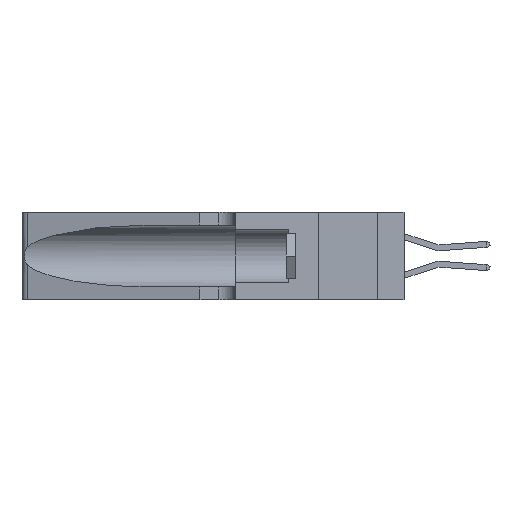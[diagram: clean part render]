
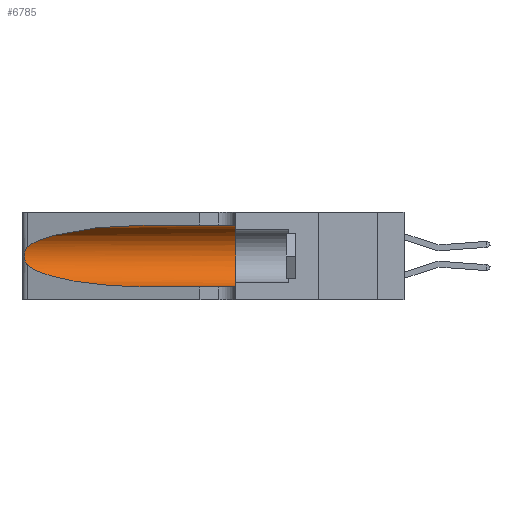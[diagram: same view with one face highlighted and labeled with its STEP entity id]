
A CAD part, left-side view. The second image highlights one B-rep face of the part: STEP entity #6785.
In plain terms, the highlighted cylindrical face has radius 3.308 mm (diameter 6.617 mm), a partial arc.
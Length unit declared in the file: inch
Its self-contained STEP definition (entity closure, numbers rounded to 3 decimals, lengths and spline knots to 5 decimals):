
#809 = ORIENTED_EDGE ( 'NONE', *, *, #11484, .T. ) ;
#860 = CARTESIAN_POINT ( 'NONE',  ( 0.1305, 0.35, 0.05475 ) ) ;
#957 = ORIENTED_EDGE ( 'NONE', *, *, #4962, .T. ) ;
#992 = DIRECTION ( 'NONE',  ( 0., -1., 0. ) ) ;
#998 = VERTEX_POINT ( 'NONE', #6603 ) ;
#1192 = DIRECTION ( 'NONE',  ( 0., 0., 1. ) ) ;
#1731 = EDGE_CURVE ( 'NONE', #15621, #19204, #7611, .T. ) ;
#1998 = CARTESIAN_POINT ( 'NONE',  ( 0.25856, 1.23593, 0.16098 ) ) ;
#2071 = CARTESIAN_POINT ( 'NONE',  ( 0.26017, 1.23833, 0.17102 ) ) ;
#2073 = CARTESIAN_POINT ( 'NONE',  ( 0.1305, 0.35, 0.31525 ) ) ;
#2075 = VECTOR ( 'NONE', #992, 39.37008 ) ;
#3475 = CARTESIAN_POINT ( 'NONE',  ( 0.26075, 1.23896, 0.19203 ) ) ;
#3716 = DIRECTION ( 'NONE',  ( 0., 0., -1. ) ) ;
#3775 =( BOUNDED_CURVE ( )  B_SPLINE_CURVE ( 3, ( #13811, #8723, #13884, #8655 ),
 .UNSPECIFIED., .F., .F. ) 
 B_SPLINE_CURVE_WITH_KNOTS ( ( 4, 4 ),
 ( 3.44316, 4.71239 ),
 .UNSPECIFIED. ) 
 CURVE ( )  GEOMETRIC_REPRESENTATION_ITEM ( )  RATIONAL_B_SPLINE_CURVE ( ( 1., 0.87, 0.87, 1. ) ) 
 REPRESENTATION_ITEM ( '' )  );
#4962 = EDGE_CURVE ( 'NONE', #17491, #6779, #10878, .T. ) ;
#5214 = FACE_OUTER_BOUND ( 'NONE', #16235, .T. ) ;
#5416 = CARTESIAN_POINT ( 'NONE',  ( 0.1305, 0.72297, 0.31525 ) ) ;
#6315 = CARTESIAN_POINT ( 'NONE',  ( 0.1305, 0.72297, 0.31525 ) ) ;
#6603 = CARTESIAN_POINT ( 'NONE',  ( 0.1305, 0.72297, 0.05475 ) ) ;
#6779 = VERTEX_POINT ( 'NONE', #15346 ) ;
#6785 = ADVANCED_FACE ( 'NONE', ( #5214 ), #8625, .F. ) ;
#6933 = CARTESIAN_POINT ( 'NONE',  ( 0.25555, 1.22993, 0.14849 ) ) ;
#7284 =( BOUNDED_CURVE ( )  B_SPLINE_CURVE ( 3, ( #6315, #8002, #19713, #18165 ),
 .UNSPECIFIED., .F., .F. ) 
 B_SPLINE_CURVE_WITH_KNOTS ( ( 4, 4 ),
 ( 1.5708, 2.84003 ),
 .UNSPECIFIED. ) 
 CURVE ( )  GEOMETRIC_REPRESENTATION_ITEM ( )  RATIONAL_B_SPLINE_CURVE ( ( 1., 0.87, 0.87, 1. ) ) 
 REPRESENTATION_ITEM ( '' )  );
#7611 = LINE ( 'NONE', #7691, #2075 ) ;
#7691 = CARTESIAN_POINT ( 'NONE',  ( 0.1305, 1.61858, 0.31525 ) ) ;
#7923 = EDGE_CURVE ( 'NONE', #19204, #19165, #18808, .T. ) ;
#8002 = CARTESIAN_POINT ( 'NONE',  ( 0.18966, 0.96281, 0.31525 ) ) ;
#8556 = CARTESIAN_POINT ( 'NONE',  ( 0.25787, 1.23484, 0.2124 ) ) ;
#8625 = CYLINDRICAL_SURFACE ( 'NONE', #14839, 0.13025 ) ;
#8655 = CARTESIAN_POINT ( 'NONE',  ( 0.1305, 0.72297, 0.05475 ) ) ;
#8723 = CARTESIAN_POINT ( 'NONE',  ( 0.2373, 1.15595, 0.08982 ) ) ;
#8931 = DIRECTION ( 'NONE',  ( 0., -1., 0. ) ) ;
#9776 = DIRECTION ( 'NONE',  ( 0., 1., 0. ) ) ;
#10351 = CARTESIAN_POINT ( 'NONE',  ( 0.25487, 1.22718, 0.22369 ) ) ;
#10504 = CARTESIAN_POINT ( 'NONE',  ( 0.1305, 1.61858, 0.185 ) ) ;
#10632 = VECTOR ( 'NONE', #18409, 39.37008 ) ;
#10878 = B_SPLINE_CURVE_WITH_KNOTS ( 'NONE', 3,
 ( #10351, #12099, #20464, #8556, #13638, #18496, #3475, #18569, #2071, #1998, #15399, #18716, #6933, #13564 ),
 .UNSPECIFIED., .F., .F.,
 ( 4, 2, 2, 2, 2, 2, 4 ),
 ( 0., 0.00027, 0.00053, 0.00107, 0.0016, 0.00187, 0.00214 ),
 .UNSPECIFIED. ) ;
#11484 = EDGE_CURVE ( 'NONE', #998, #19165, #13755, .T. ) ;
#11628 = ORIENTED_EDGE ( 'NONE', *, *, #12386, .T. ) ;
#12099 = CARTESIAN_POINT ( 'NONE',  ( 0.25555, 1.22994, 0.2215 ) ) ;
#12386 = EDGE_CURVE ( 'NONE', #15621, #17491, #7284, .T. ) ;
#13564 = CARTESIAN_POINT ( 'NONE',  ( 0.25487, 1.22718, 0.14631 ) ) ;
#13638 = CARTESIAN_POINT ( 'NONE',  ( 0.25854, 1.2359, 0.20912 ) ) ;
#13755 = LINE ( 'NONE', #14954, #10632 ) ;
#13811 = CARTESIAN_POINT ( 'NONE',  ( 0.25487, 1.22718, 0.14631 ) ) ;
#13884 = CARTESIAN_POINT ( 'NONE',  ( 0.18966, 0.96281, 0.05475 ) ) ;
#14345 = EDGE_CURVE ( 'NONE', #6779, #998, #3775, .T. ) ;
#14361 = ORIENTED_EDGE ( 'NONE', *, *, #1731, .F. ) ;
#14839 = AXIS2_PLACEMENT_3D ( 'NONE', #10504, #8931, #3716 ) ;
#14880 = CARTESIAN_POINT ( 'NONE',  ( 0.25487, 1.22718, 0.22369 ) ) ;
#14954 = CARTESIAN_POINT ( 'NONE',  ( 0.1305, 1.61858, 0.05475 ) ) ;
#15346 = CARTESIAN_POINT ( 'NONE',  ( 0.25487, 1.22718, 0.14631 ) ) ;
#15399 = CARTESIAN_POINT ( 'NONE',  ( 0.25789, 1.23486, 0.15765 ) ) ;
#15621 = VERTEX_POINT ( 'NONE', #5416 ) ;
#16148 = AXIS2_PLACEMENT_3D ( 'NONE', #19811, #9776, #1192 ) ;
#16235 = EDGE_LOOP ( 'NONE', ( #11628, #957, #21155, #809, #17422, #14361 ) ) ;
#17422 = ORIENTED_EDGE ( 'NONE', *, *, #7923, .F. ) ;
#17491 = VERTEX_POINT ( 'NONE', #14880 ) ;
#18165 = CARTESIAN_POINT ( 'NONE',  ( 0.25487, 1.22718, 0.22369 ) ) ;
#18409 = DIRECTION ( 'NONE',  ( 0., -1., 0. ) ) ;
#18496 = CARTESIAN_POINT ( 'NONE',  ( 0.26018, 1.23835, 0.19895 ) ) ;
#18569 = CARTESIAN_POINT ( 'NONE',  ( 0.26075, 1.23896, 0.178 ) ) ;
#18716 = CARTESIAN_POINT ( 'NONE',  ( 0.25639, 1.23186, 0.15144 ) ) ;
#18808 = CIRCLE ( 'NONE', #16148, 0.13025 ) ;
#19165 = VERTEX_POINT ( 'NONE', #860 ) ;
#19204 = VERTEX_POINT ( 'NONE', #2073 ) ;
#19713 = CARTESIAN_POINT ( 'NONE',  ( 0.2373, 1.15595, 0.28018 ) ) ;
#19811 = CARTESIAN_POINT ( 'NONE',  ( 0.1305, 0.35, 0.185 ) ) ;
#20464 = CARTESIAN_POINT ( 'NONE',  ( 0.25639, 1.23184, 0.21858 ) ) ;
#21155 = ORIENTED_EDGE ( 'NONE', *, *, #14345, .T. ) ;
